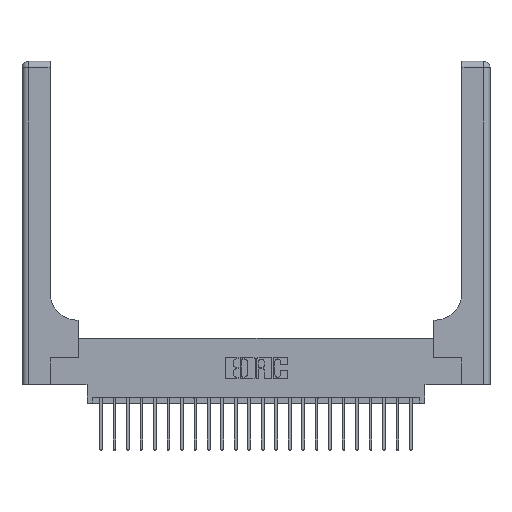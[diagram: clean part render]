
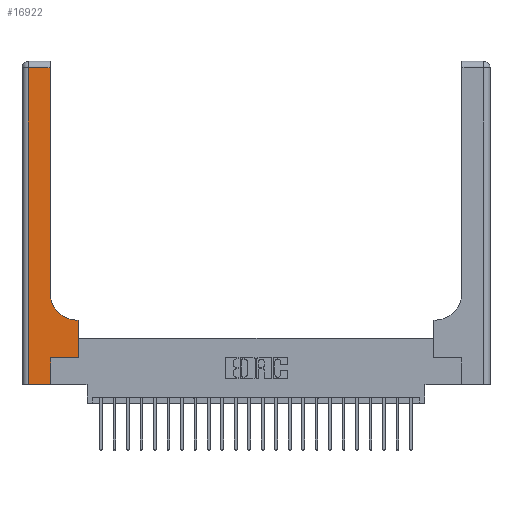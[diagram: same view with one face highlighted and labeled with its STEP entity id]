
A CAD part, top view. The second image highlights one B-rep face of the part: STEP entity #16922.
In plain terms, the highlighted planar face has unit normal (0, 0, 1).
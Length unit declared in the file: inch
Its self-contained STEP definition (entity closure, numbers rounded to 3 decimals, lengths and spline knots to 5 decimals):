
#337 = EDGE_CURVE ( 'NONE', #22943, #19265, #3038, .T. ) ;
#815 = LINE ( 'NONE', #8185, #18328 ) ;
#883 = DIRECTION ( 'NONE',  ( 0., 1., 0. ) ) ;
#1299 = DIRECTION ( 'NONE',  ( -1., 0., 0. ) ) ;
#2416 = CARTESIAN_POINT ( 'NONE',  ( 0.528, 0.25, 0.37 ) ) ;
#2447 = DIRECTION ( 'NONE',  ( 1., 0., 0. ) ) ;
#2831 = EDGE_CURVE ( 'NONE', #3562, #16256, #10140, .T. ) ;
#2842 = VECTOR ( 'NONE', #1299, 39.37008 ) ;
#3038 = LINE ( 'NONE', #17744, #15421 ) ;
#3341 = CARTESIAN_POINT ( 'NONE',  ( 0., 3., 0.37 ) ) ;
#3562 = VERTEX_POINT ( 'NONE', #10820 ) ;
#3585 = VECTOR ( 'NONE', #883, 39.37008 ) ;
#3784 = VERTEX_POINT ( 'NONE', #6199 ) ;
#3859 = CARTESIAN_POINT ( 'NONE',  ( 0., 0., 0.37 ) ) ;
#3972 = VECTOR ( 'NONE', #11240, 39.37008 ) ;
#4003 = ORIENTED_EDGE ( 'NONE', *, *, #337, .T. ) ;
#4269 = VECTOR ( 'NONE', #5039, 39.37008 ) ;
#4559 = VERTEX_POINT ( 'NONE', #21090 ) ;
#5039 = DIRECTION ( 'NONE',  ( 1., 0., 0. ) ) ;
#5076 = CIRCLE ( 'NONE', #6611, 0.25 ) ;
#6053 = DIRECTION ( 'NONE',  ( 0., 1., 0. ) ) ;
#6088 = DIRECTION ( 'NONE',  ( 0., 0., -1. ) ) ;
#6199 = CARTESIAN_POINT ( 'NONE',  ( 0.265, 0.25, 0.37 ) ) ;
#6380 = ORIENTED_EDGE ( 'NONE', *, *, #21520, .T. ) ;
#6611 = AXIS2_PLACEMENT_3D ( 'NONE', #15240, #6088, #2447 ) ;
#6631 = EDGE_LOOP ( 'NONE', ( #7491, #15014, #17081, #22060, #6380, #7934, #14747, #4003, #21283 ) ) ;
#6660 = EDGE_CURVE ( 'NONE', #12650, #20813, #23799, .T. ) ;
#7319 = EDGE_CURVE ( 'NONE', #17246, #3562, #815, .T. ) ;
#7491 = ORIENTED_EDGE ( 'NONE', *, *, #7319, .T. ) ;
#7934 = ORIENTED_EDGE ( 'NONE', *, *, #12912, .T. ) ;
#8185 = CARTESIAN_POINT ( 'NONE',  ( 0.26, 3., 0.37 ) ) ;
#8251 = CARTESIAN_POINT ( 'NONE',  ( 0.265, 0., 0.37 ) ) ;
#9377 = CARTESIAN_POINT ( 'NONE',  ( 0.265, 0., 0.37 ) ) ;
#10140 = LINE ( 'NONE', #21356, #2842 ) ;
#10273 = EDGE_CURVE ( 'NONE', #16256, #12650, #12153, .T. ) ;
#10820 = CARTESIAN_POINT ( 'NONE',  ( 0.26, 2.94, 0.37 ) ) ;
#11162 = CARTESIAN_POINT ( 'NONE',  ( 0.06, 2.94, 0.37 ) ) ;
#11193 = DIRECTION ( 'NONE',  ( -1., 0., 0. ) ) ;
#11197 = VECTOR ( 'NONE', #6053, 39.37008 ) ;
#11240 = DIRECTION ( 'NONE',  ( 1., 0., 0. ) ) ;
#12032 = DIRECTION ( 'NONE',  ( 0., -1., 0. ) ) ;
#12146 = EDGE_CURVE ( 'NONE', #4559, #22943, #18832, .T. ) ;
#12153 = LINE ( 'NONE', #13723, #14654 ) ;
#12650 = VERTEX_POINT ( 'NONE', #13157 ) ;
#12873 = DIRECTION ( 'NONE',  ( 0., 1., 0. ) ) ;
#12912 = EDGE_CURVE ( 'NONE', #3784, #4559, #16017, .T. ) ;
#13157 = CARTESIAN_POINT ( 'NONE',  ( 0.06, 0., 0.37 ) ) ;
#13720 = EDGE_CURVE ( 'NONE', #19265, #17246, #5076, .T. ) ;
#13723 = CARTESIAN_POINT ( 'NONE',  ( 0.06, 3., 0.37 ) ) ;
#14279 = LINE ( 'NONE', #8251, #3585 ) ;
#14290 = AXIS2_PLACEMENT_3D ( 'NONE', #3341, #23861, #11193 ) ;
#14654 = VECTOR ( 'NONE', #12032, 39.37008 ) ;
#14747 = ORIENTED_EDGE ( 'NONE', *, *, #12146, .T. ) ;
#15014 = ORIENTED_EDGE ( 'NONE', *, *, #2831, .T. ) ;
#15240 = CARTESIAN_POINT ( 'NONE',  ( 0.51, 0.85, 0.37 ) ) ;
#15421 = VECTOR ( 'NONE', #16758, 39.37008 ) ;
#15874 = CARTESIAN_POINT ( 'NONE',  ( 0.26, 0.85, 0.37 ) ) ;
#16017 = LINE ( 'NONE', #21720, #4269 ) ;
#16256 = VERTEX_POINT ( 'NONE', #11162 ) ;
#16758 = DIRECTION ( 'NONE',  ( -1., 0., 0. ) ) ;
#16922 = ADVANCED_FACE ( 'NONE', ( #18051 ), #19883, .F. ) ;
#17081 = ORIENTED_EDGE ( 'NONE', *, *, #10273, .T. ) ;
#17246 = VERTEX_POINT ( 'NONE', #15874 ) ;
#17744 = CARTESIAN_POINT ( 'NONE',  ( 0.26, 0.6, 0.37 ) ) ;
#18051 = FACE_OUTER_BOUND ( 'NONE', #6631, .T. ) ;
#18328 = VECTOR ( 'NONE', #12873, 39.37008 ) ;
#18832 = LINE ( 'NONE', #2416, #11197 ) ;
#19265 = VERTEX_POINT ( 'NONE', #20864 ) ;
#19883 = PLANE ( 'NONE',  #14290 ) ;
#20813 = VERTEX_POINT ( 'NONE', #9377 ) ;
#20864 = CARTESIAN_POINT ( 'NONE',  ( 0.51, 0.6, 0.37 ) ) ;
#21090 = CARTESIAN_POINT ( 'NONE',  ( 0.528, 0.25, 0.37 ) ) ;
#21283 = ORIENTED_EDGE ( 'NONE', *, *, #13720, .T. ) ;
#21356 = CARTESIAN_POINT ( 'NONE',  ( 0., 2.94, 0.37 ) ) ;
#21520 = EDGE_CURVE ( 'NONE', #20813, #3784, #14279, .T. ) ;
#21720 = CARTESIAN_POINT ( 'NONE',  ( 0.265, 0.25, 0.37 ) ) ;
#22060 = ORIENTED_EDGE ( 'NONE', *, *, #6660, .T. ) ;
#22694 = CARTESIAN_POINT ( 'NONE',  ( 0.528, 0.6, 0.37 ) ) ;
#22943 = VERTEX_POINT ( 'NONE', #22694 ) ;
#23799 = LINE ( 'NONE', #3859, #3972 ) ;
#23861 = DIRECTION ( 'NONE',  ( 0., 0., -1. ) ) ;
